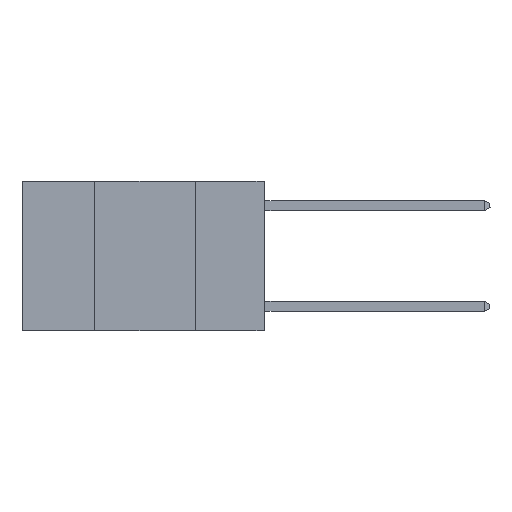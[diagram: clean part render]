
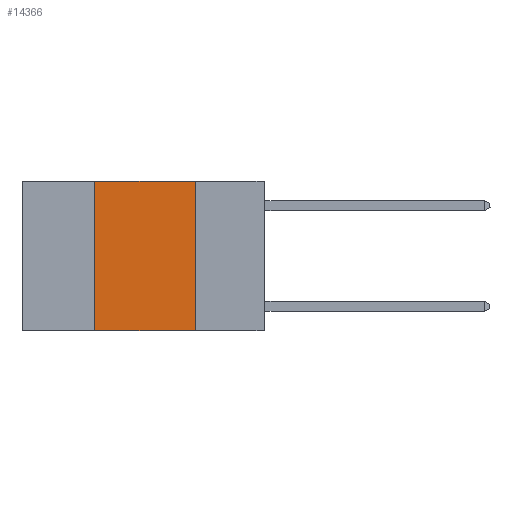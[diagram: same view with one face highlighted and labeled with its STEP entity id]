
A CAD part, left-side view. The second image highlights one B-rep face of the part: STEP entity #14366.
In plain terms, the highlighted planar face has unit normal (-1, 0, 0).
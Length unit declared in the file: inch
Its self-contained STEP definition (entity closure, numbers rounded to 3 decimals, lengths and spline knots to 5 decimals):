
#356 = FACE_OUTER_BOUND ( 'NONE', #777, .T. ) ;
#554 = CARTESIAN_POINT ( 'NONE',  ( 0., 0.42, 0. ) ) ;
#777 = EDGE_LOOP ( 'NONE', ( #4946, #9192, #7793, #1596 ) ) ;
#1596 = ORIENTED_EDGE ( 'NONE', *, *, #12602, .T. ) ;
#1828 = LINE ( 'NONE', #6356, #4857 ) ;
#1842 = AXIS2_PLACEMENT_3D ( 'NONE', #10920, #5306, #13145 ) ;
#1959 = CARTESIAN_POINT ( 'NONE',  ( 0., 0.6, 0. ) ) ;
#2279 = CARTESIAN_POINT ( 'NONE',  ( 0., 0.42, -0.37 ) ) ;
#2378 = VECTOR ( 'NONE', #6513, 39.37008 ) ;
#3071 = CARTESIAN_POINT ( 'NONE',  ( 0., 0.42, 0. ) ) ;
#3696 = VERTEX_POINT ( 'NONE', #12316 ) ;
#4717 = LINE ( 'NONE', #3071, #13341 ) ;
#4857 = VECTOR ( 'NONE', #7491, 39.37008 ) ;
#4946 = ORIENTED_EDGE ( 'NONE', *, *, #7415, .F. ) ;
#5306 = DIRECTION ( 'NONE',  ( 1., 0., 0. ) ) ;
#6356 = CARTESIAN_POINT ( 'NONE',  ( 0., 0.17, 0. ) ) ;
#6513 = DIRECTION ( 'NONE',  ( 0., -1., 0. ) ) ;
#7112 = VERTEX_POINT ( 'NONE', #2279 ) ;
#7415 = EDGE_CURVE ( 'NONE', #10876, #3696, #1828, .T. ) ;
#7491 = DIRECTION ( 'NONE',  ( 0., 0., -1. ) ) ;
#7793 = ORIENTED_EDGE ( 'NONE', *, *, #12198, .F. ) ;
#8199 = EDGE_CURVE ( 'NONE', #13797, #10876, #11547, .T. ) ;
#8568 = VECTOR ( 'NONE', #12163, 39.37008 ) ;
#8589 = CARTESIAN_POINT ( 'NONE',  ( 0., 0.17, 0. ) ) ;
#8749 = CARTESIAN_POINT ( 'NONE',  ( 0., 0.6, -0.37 ) ) ;
#8796 = DIRECTION ( 'NONE',  ( 0., 0., 1. ) ) ;
#9192 = ORIENTED_EDGE ( 'NONE', *, *, #8199, .F. ) ;
#9799 = PLANE ( 'NONE',  #1842 ) ;
#10876 = VERTEX_POINT ( 'NONE', #8589 ) ;
#10920 = CARTESIAN_POINT ( 'NONE',  ( 0., 0.6, 0. ) ) ;
#11082 = LINE ( 'NONE', #8749, #2378 ) ;
#11547 = LINE ( 'NONE', #1959, #8568 ) ;
#12163 = DIRECTION ( 'NONE',  ( 0., -1., 0. ) ) ;
#12198 = EDGE_CURVE ( 'NONE', #7112, #13797, #4717, .T. ) ;
#12316 = CARTESIAN_POINT ( 'NONE',  ( 0., 0.17, -0.37 ) ) ;
#12602 = EDGE_CURVE ( 'NONE', #7112, #3696, #11082, .T. ) ;
#13145 = DIRECTION ( 'NONE',  ( 0., 0., -1. ) ) ;
#13341 = VECTOR ( 'NONE', #8796, 39.37008 ) ;
#13797 = VERTEX_POINT ( 'NONE', #554 ) ;
#14366 = ADVANCED_FACE ( 'NONE', ( #356 ), #9799, .F. ) ;
